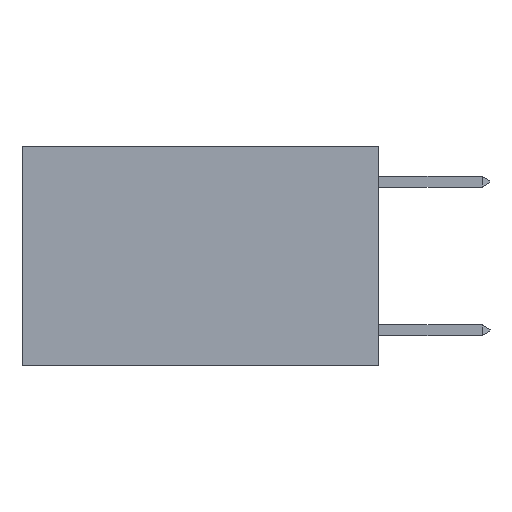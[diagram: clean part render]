
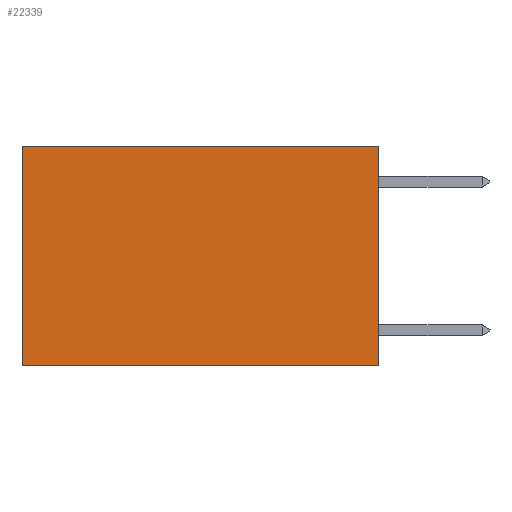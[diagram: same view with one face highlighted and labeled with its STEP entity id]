
A CAD part, left-side view. The second image highlights one B-rep face of the part: STEP entity #22339.
In plain terms, the highlighted planar face has unit normal (-1, 0, 0).
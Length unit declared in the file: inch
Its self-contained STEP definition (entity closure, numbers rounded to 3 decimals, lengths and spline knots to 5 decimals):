
#367 = CARTESIAN_POINT ( 'NONE',  ( 0.2625, 0., 0. ) ) ;
#676 = AXIS2_PLACEMENT_3D ( 'NONE', #7062, #8946, #21411 ) ;
#1477 = VERTEX_POINT ( 'NONE', #8261 ) ;
#1643 = VERTEX_POINT ( 'NONE', #15970 ) ;
#3002 = DIRECTION ( 'NONE',  ( 0., 1., 0. ) ) ;
#3006 = CARTESIAN_POINT ( 'NONE',  ( 0.2625, 0.6, 0. ) ) ;
#4229 = DIRECTION ( 'NONE',  ( 0., 0., -1. ) ) ;
#4354 = VECTOR ( 'NONE', #15441, 39.37008 ) ;
#4827 = VECTOR ( 'NONE', #4229, 39.37008 ) ;
#5145 = PLANE ( 'NONE',  #676 ) ;
#5709 = ORIENTED_EDGE ( 'NONE', *, *, #13551, .T. ) ;
#7062 = CARTESIAN_POINT ( 'NONE',  ( 0.2625, 0., 0. ) ) ;
#8261 = CARTESIAN_POINT ( 'NONE',  ( 0.2625, 0., -0.37 ) ) ;
#8946 = DIRECTION ( 'NONE',  ( 1., 0., 0. ) ) ;
#9390 = EDGE_CURVE ( 'NONE', #22293, #19950, #18332, .T. ) ;
#9855 = LINE ( 'NONE', #367, #4827 ) ;
#11117 = ORIENTED_EDGE ( 'NONE', *, *, #9390, .T. ) ;
#12078 = EDGE_CURVE ( 'NONE', #1643, #1477, #9855, .T. ) ;
#12253 = CARTESIAN_POINT ( 'NONE',  ( 0.2625, 0., -0.37 ) ) ;
#12628 = VECTOR ( 'NONE', #13973, 39.37008 ) ;
#13221 = VECTOR ( 'NONE', #3002, 39.37008 ) ;
#13551 = EDGE_CURVE ( 'NONE', #1643, #22293, #21499, .T. ) ;
#13973 = DIRECTION ( 'NONE',  ( 0., 1., 0. ) ) ;
#14281 = ORIENTED_EDGE ( 'NONE', *, *, #23574, .F. ) ;
#14437 = EDGE_LOOP ( 'NONE', ( #11117, #14281, #16653, #5709 ) ) ;
#15441 = DIRECTION ( 'NONE',  ( 0., 0., -1. ) ) ;
#15970 = CARTESIAN_POINT ( 'NONE',  ( 0.2625, 0., 0. ) ) ;
#16653 = ORIENTED_EDGE ( 'NONE', *, *, #12078, .F. ) ;
#17612 = CARTESIAN_POINT ( 'NONE',  ( 0.2625, 0., 0. ) ) ;
#17961 = LINE ( 'NONE', #12253, #13221 ) ;
#18332 = LINE ( 'NONE', #22139, #4354 ) ;
#18544 = CARTESIAN_POINT ( 'NONE',  ( 0.2625, 0.6, -0.37 ) ) ;
#19950 = VERTEX_POINT ( 'NONE', #18544 ) ;
#20497 = FACE_OUTER_BOUND ( 'NONE', #14437, .T. ) ;
#21411 = DIRECTION ( 'NONE',  ( 0., 0., -1. ) ) ;
#21499 = LINE ( 'NONE', #17612, #12628 ) ;
#22139 = CARTESIAN_POINT ( 'NONE',  ( 0.2625, 0.6, 0. ) ) ;
#22293 = VERTEX_POINT ( 'NONE', #3006 ) ;
#22339 = ADVANCED_FACE ( 'NONE', ( #20497 ), #5145, .F. ) ;
#23574 = EDGE_CURVE ( 'NONE', #1477, #19950, #17961, .T. ) ;
